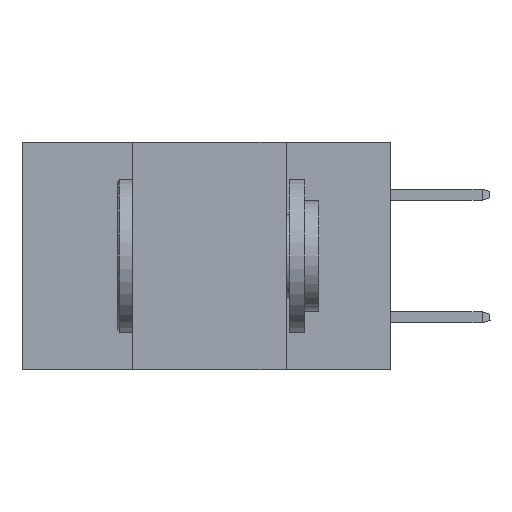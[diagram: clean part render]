
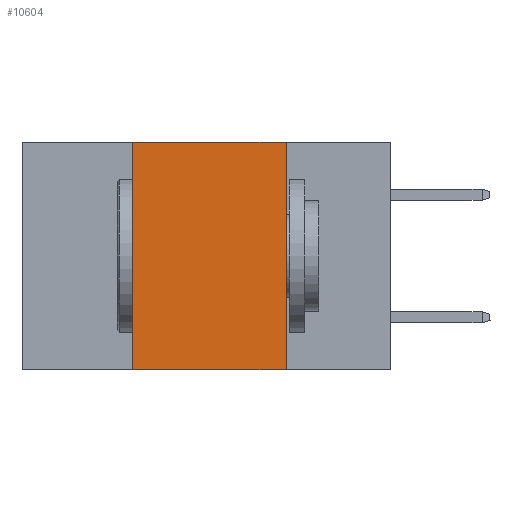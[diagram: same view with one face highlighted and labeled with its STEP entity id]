
A CAD part, left-side view. The second image highlights one B-rep face of the part: STEP entity #10604.
In plain terms, the highlighted planar face has unit normal (-1, 0, 0).
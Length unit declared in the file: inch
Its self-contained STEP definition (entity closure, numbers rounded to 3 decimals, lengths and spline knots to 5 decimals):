
#90 = CARTESIAN_POINT ( 'NONE',  ( 0., 0.6, 0. ) ) ;
#1174 = ORIENTED_EDGE ( 'NONE', *, *, #2225, .F. ) ;
#2225 = EDGE_CURVE ( 'NONE', #14279, #2257, #16524, .T. ) ;
#2257 = VERTEX_POINT ( 'NONE', #7322 ) ;
#2275 = VERTEX_POINT ( 'NONE', #9879 ) ;
#3258 = DIRECTION ( 'NONE',  ( 1., 0., 0. ) ) ;
#5308 = AXIS2_PLACEMENT_3D ( 'NONE', #12499, #3258, #5957 ) ;
#5795 = FACE_OUTER_BOUND ( 'NONE', #7630, .T. ) ;
#5942 = ORIENTED_EDGE ( 'NONE', *, *, #6726, .T. ) ;
#5957 = DIRECTION ( 'NONE',  ( 0., 0., -1. ) ) ;
#6131 = LINE ( 'NONE', #9349, #15154 ) ;
#6141 = ORIENTED_EDGE ( 'NONE', *, *, #11782, .F. ) ;
#6726 = EDGE_CURVE ( 'NONE', #7193, #2257, #6131, .T. ) ;
#7193 = VERTEX_POINT ( 'NONE', #16608 ) ;
#7322 = CARTESIAN_POINT ( 'NONE',  ( 0., 0.17, -0.37 ) ) ;
#7630 = EDGE_LOOP ( 'NONE', ( #1174, #6141, #15449, #5942 ) ) ;
#8799 = CARTESIAN_POINT ( 'NONE',  ( 0., 0.42, 0. ) ) ;
#9249 = VECTOR ( 'NONE', #11690, 39.37008 ) ;
#9349 = CARTESIAN_POINT ( 'NONE',  ( 0., 0.6, -0.37 ) ) ;
#9549 = VECTOR ( 'NONE', #15043, 39.37008 ) ;
#9879 = CARTESIAN_POINT ( 'NONE',  ( 0., 0.42, 0. ) ) ;
#10138 = DIRECTION ( 'NONE',  ( 0., -1., 0. ) ) ;
#10604 = ADVANCED_FACE ( 'NONE', ( #5795 ), #13813, .F. ) ;
#10676 = LINE ( 'NONE', #8799, #9249 ) ;
#10858 = LINE ( 'NONE', #90, #15599 ) ;
#11690 = DIRECTION ( 'NONE',  ( 0., 0., 1. ) ) ;
#11782 = EDGE_CURVE ( 'NONE', #2275, #14279, #10858, .T. ) ;
#12499 = CARTESIAN_POINT ( 'NONE',  ( 0., 0.6, 0. ) ) ;
#13771 = CARTESIAN_POINT ( 'NONE',  ( 0., 0.17, 0. ) ) ;
#13813 = PLANE ( 'NONE',  #5308 ) ;
#14279 = VERTEX_POINT ( 'NONE', #15196 ) ;
#14516 = DIRECTION ( 'NONE',  ( 0., -1., 0. ) ) ;
#14926 = EDGE_CURVE ( 'NONE', #7193, #2275, #10676, .T. ) ;
#15043 = DIRECTION ( 'NONE',  ( 0., 0., -1. ) ) ;
#15154 = VECTOR ( 'NONE', #10138, 39.37008 ) ;
#15196 = CARTESIAN_POINT ( 'NONE',  ( 0., 0.17, 0. ) ) ;
#15449 = ORIENTED_EDGE ( 'NONE', *, *, #14926, .F. ) ;
#15599 = VECTOR ( 'NONE', #14516, 39.37008 ) ;
#16524 = LINE ( 'NONE', #13771, #9549 ) ;
#16608 = CARTESIAN_POINT ( 'NONE',  ( 0., 0.42, -0.37 ) ) ;
